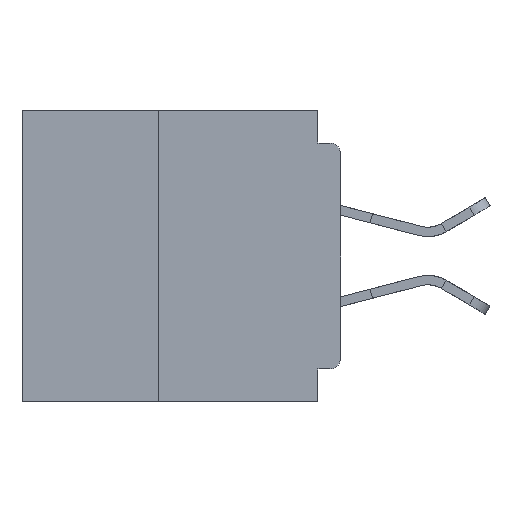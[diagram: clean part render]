
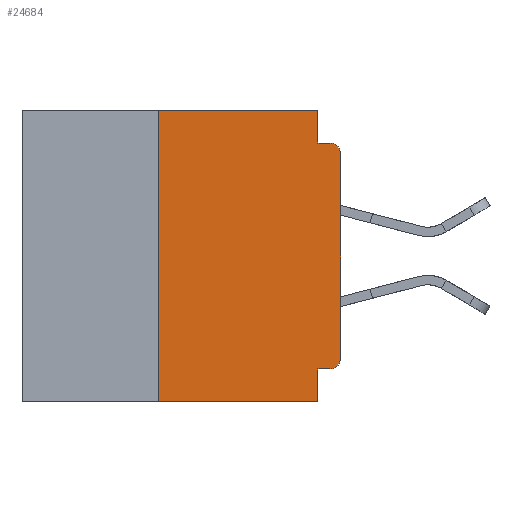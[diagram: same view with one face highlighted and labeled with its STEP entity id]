
A CAD part, left-side view. The second image highlights one B-rep face of the part: STEP entity #24684.
In plain terms, the highlighted planar face has unit normal (-1, 0, 0).
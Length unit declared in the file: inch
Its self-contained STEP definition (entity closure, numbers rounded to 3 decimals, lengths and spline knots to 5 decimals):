
#504 = EDGE_CURVE ( 'NONE', #14713, #5673, #28726, .T. ) ;
#1005 = CARTESIAN_POINT ( 'NONE',  ( 0., 0.015, -0.34 ) ) ;
#1014 = ORIENTED_EDGE ( 'NONE', *, *, #37631, .T. ) ;
#1036 = LINE ( 'NONE', #35671, #36099 ) ;
#1091 = ORIENTED_EDGE ( 'NONE', *, *, #9794, .T. ) ;
#1556 = ORIENTED_EDGE ( 'NONE', *, *, #27730, .F. ) ;
#1643 = ORIENTED_EDGE ( 'NONE', *, *, #2920, .F. ) ;
#2037 = ORIENTED_EDGE ( 'NONE', *, *, #13175, .F. ) ;
#2069 = ORIENTED_EDGE ( 'NONE', *, *, #17637, .F. ) ;
#2084 = LINE ( 'NONE', #25788, #36094 ) ;
#2768 = ORIENTED_EDGE ( 'NONE', *, *, #21479, .T. ) ;
#2920 = EDGE_CURVE ( 'NONE', #26727, #7243, #30990, .T. ) ;
#2948 = ORIENTED_EDGE ( 'NONE', *, *, #504, .F. ) ;
#3094 = AXIS2_PLACEMENT_3D ( 'NONE', #1005, #24136, #4345 ) ;
#3424 = ORIENTED_EDGE ( 'NONE', *, *, #10722, .F. ) ;
#3579 = ORIENTED_EDGE ( 'NONE', *, *, #3791, .T. ) ;
#3791 = EDGE_CURVE ( 'NONE', #19534, #15457, #30909, .T. ) ;
#3841 = CARTESIAN_POINT ( 'NONE',  ( 0., 0.015, -0.06 ) ) ;
#4312 = CARTESIAN_POINT ( 'NONE',  ( 0., 0.031, -0.4 ) ) ;
#4345 = DIRECTION ( 'NONE',  ( 0., 0., -1. ) ) ;
#4700 = VECTOR ( 'NONE', #31529, 39.37008 ) ;
#5413 = FACE_OUTER_BOUND ( 'NONE', #28427, .T. ) ;
#5673 = VERTEX_POINT ( 'NONE', #14330 ) ;
#6245 = DIRECTION ( 'NONE',  ( 0., 0., -1. ) ) ;
#7173 = DIRECTION ( 'NONE',  ( 0., 0., -1. ) ) ;
#7243 = VERTEX_POINT ( 'NONE', #27251 ) ;
#7604 = AXIS2_PLACEMENT_3D ( 'NONE', #22741, #26013, #6245 ) ;
#8731 = CARTESIAN_POINT ( 'NONE',  ( 0., 0., -0.355 ) ) ;
#8927 = DIRECTION ( 'NONE',  ( 0., 0., -1. ) ) ;
#9316 = CARTESIAN_POINT ( 'NONE',  ( 0., 0., -0.34 ) ) ;
#9794 = EDGE_CURVE ( 'NONE', #37401, #16794, #12175, .T. ) ;
#10722 = EDGE_CURVE ( 'NONE', #19534, #14713, #36826, .T. ) ;
#11348 = AXIS2_PLACEMENT_3D ( 'NONE', #3841, #26919, #7173 ) ;
#12175 = CIRCLE ( 'NONE', #11348, 0.015 ) ;
#12644 = VECTOR ( 'NONE', #34020, 39.37008 ) ;
#12904 = DIRECTION ( 'NONE',  ( 0., 0., 1. ) ) ;
#13175 = EDGE_CURVE ( 'NONE', #33083, #26727, #1036, .T. ) ;
#14330 = CARTESIAN_POINT ( 'NONE',  ( 0., 0.031, -0.4 ) ) ;
#14713 = VERTEX_POINT ( 'NONE', #27366 ) ;
#15457 = VERTEX_POINT ( 'NONE', #9316 ) ;
#15981 = DIRECTION ( 'NONE',  ( 0., -1., 0. ) ) ;
#16794 = VERTEX_POINT ( 'NONE', #29882 ) ;
#17637 = EDGE_CURVE ( 'NONE', #26296, #33083, #36251, .T. ) ;
#17985 = CARTESIAN_POINT ( 'NONE',  ( 0., 0.015, -0.355 ) ) ;
#19371 = PLANE ( 'NONE',  #7604 ) ;
#19534 = VERTEX_POINT ( 'NONE', #17985 ) ;
#20800 = CARTESIAN_POINT ( 'NONE',  ( 0., 0., -0.045 ) ) ;
#21479 = EDGE_CURVE ( 'NONE', #26296, #5673, #2084, .T. ) ;
#22600 = CARTESIAN_POINT ( 'NONE',  ( 0., 0., 0. ) ) ;
#22653 = DIRECTION ( 'NONE',  ( 0., -1., 0. ) ) ;
#22741 = CARTESIAN_POINT ( 'NONE',  ( 0., 0.437, 0. ) ) ;
#24136 = DIRECTION ( 'NONE',  ( -1., 0., 0. ) ) ;
#24684 = ADVANCED_FACE ( 'NONE', ( #5413 ), #19371, .F. ) ;
#25788 = CARTESIAN_POINT ( 'NONE',  ( 0., 0.437, -0.4 ) ) ;
#26013 = DIRECTION ( 'NONE',  ( 1., 0., 0. ) ) ;
#26296 = VERTEX_POINT ( 'NONE', #27899 ) ;
#26727 = VERTEX_POINT ( 'NONE', #35240 ) ;
#26919 = DIRECTION ( 'NONE',  ( -1., 0., 0. ) ) ;
#27070 = VECTOR ( 'NONE', #31884, 39.37008 ) ;
#27251 = CARTESIAN_POINT ( 'NONE',  ( 0., 0.031, -0.045 ) ) ;
#27366 = CARTESIAN_POINT ( 'NONE',  ( 0., 0.031, -0.355 ) ) ;
#27539 = VECTOR ( 'NONE', #31142, 39.37008 ) ;
#27730 = EDGE_CURVE ( 'NONE', #7243, #16794, #30107, .T. ) ;
#27854 = CARTESIAN_POINT ( 'NONE',  ( 0., 0.25, -0.4 ) ) ;
#27899 = CARTESIAN_POINT ( 'NONE',  ( 0., 0.25, -0.4 ) ) ;
#28172 = CARTESIAN_POINT ( 'NONE',  ( 0., 0.25, 0. ) ) ;
#28201 = CARTESIAN_POINT ( 'NONE',  ( 0., 0., -0.06 ) ) ;
#28427 = EDGE_LOOP ( 'NONE', ( #1014, #1091, #1556, #1643, #2037, #2069, #2768, #2948, #3424, #3579 ) ) ;
#28726 = LINE ( 'NONE', #4312, #41731 ) ;
#29882 = CARTESIAN_POINT ( 'NONE',  ( 0., 0.015, -0.045 ) ) ;
#30107 = LINE ( 'NONE', #20800, #12644 ) ;
#30612 = VECTOR ( 'NONE', #12904, 39.37008 ) ;
#30909 = CIRCLE ( 'NONE', #3094, 0.015 ) ;
#30990 = LINE ( 'NONE', #31710, #4700 ) ;
#31142 = DIRECTION ( 'NONE',  ( 0., 0., 1. ) ) ;
#31529 = DIRECTION ( 'NONE',  ( 0., 0., -1. ) ) ;
#31710 = CARTESIAN_POINT ( 'NONE',  ( 0., 0.031, 0. ) ) ;
#31884 = DIRECTION ( 'NONE',  ( 0., 1., 0. ) ) ;
#32685 = LINE ( 'NONE', #22600, #30612 ) ;
#33083 = VERTEX_POINT ( 'NONE', #28172 ) ;
#34020 = DIRECTION ( 'NONE',  ( 0., -1., 0. ) ) ;
#35240 = CARTESIAN_POINT ( 'NONE',  ( 0., 0.031, 0. ) ) ;
#35671 = CARTESIAN_POINT ( 'NONE',  ( 0., 0.437, 0. ) ) ;
#36094 = VECTOR ( 'NONE', #22653, 39.37008 ) ;
#36099 = VECTOR ( 'NONE', #15981, 39.37008 ) ;
#36251 = LINE ( 'NONE', #27854, #27539 ) ;
#36826 = LINE ( 'NONE', #8731, #27070 ) ;
#37401 = VERTEX_POINT ( 'NONE', #28201 ) ;
#37631 = EDGE_CURVE ( 'NONE', #15457, #37401, #32685, .T. ) ;
#41731 = VECTOR ( 'NONE', #8927, 39.37008 ) ;
